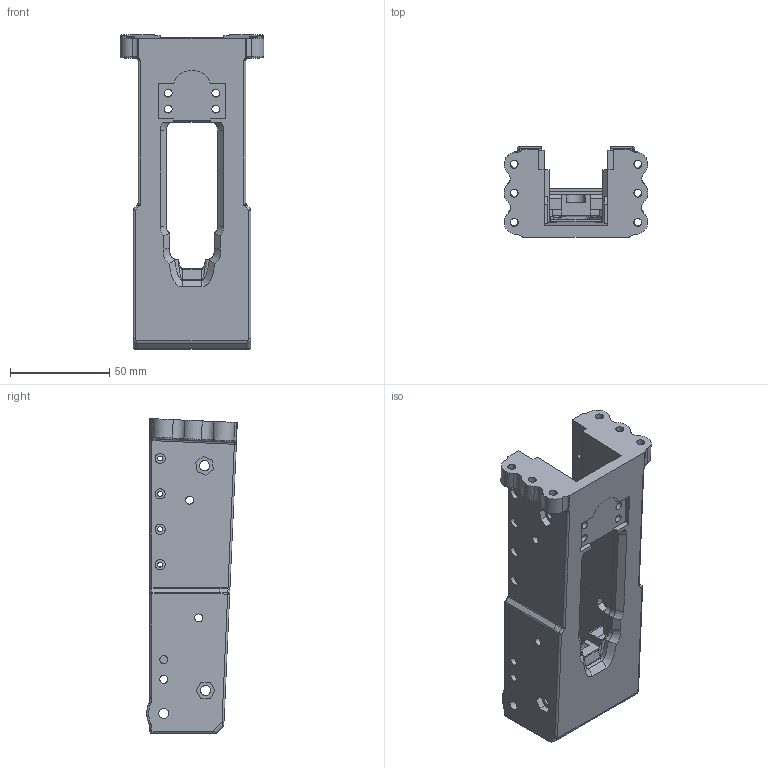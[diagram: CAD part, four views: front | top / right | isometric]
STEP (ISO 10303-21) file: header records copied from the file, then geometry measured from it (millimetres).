
FILE_DESCRIPTION(/* description */ (''),/* implementation_level */ '2;1');
FILE_NAME(/* name */ 'Plastikov v3.0 AK100-Series Front Receiver.stp',/* time_stamp */ '2022-03-22T10:43:13-05:00',/* author */ ('johne'),/* organization */ (''),/* preprocessor_version */ 'ST-DEVELOPER v18.1',/* originating_system */ 'Autodesk Inventor 2020',/* authorisation */ '');
FILE_SCHEMA (('AUTOMOTIVE_DESIGN { 1 0 10303 214 3 1 1 }'));
Length unit declared in the file: inch
Products named in the file (1): Plastikov v3.0 AK100-Series Front Receiver
Bounding box: 72.2 x 45.54 x 158.19 mm (x, y, z)
Volume: 184357.2 mm3; surface area: 47014 mm2
Topology: 1 solids, 1 shells, 376 faces, 991 edges, 620 vertices
Faces by surface type: plane 175, cylinder 117, bspline 51, torus 18, sphere 9, cone 6
Full cylindrical faces by diameter (mm): 2.5 x8, 4 x17, 5 x3, 5.08 x8, 5.1 x2, 11.989 x1, 12 x1
Entity records: 13198 total; most frequent: CARTESIAN_POINT 3850, ORIENTED_EDGE 1950, DIRECTION 1891, EDGE_CURVE 975, AXIS2_PLACEMENT_3D 662, VERTEX_POINT 620, LINE 567, VECTOR 567
